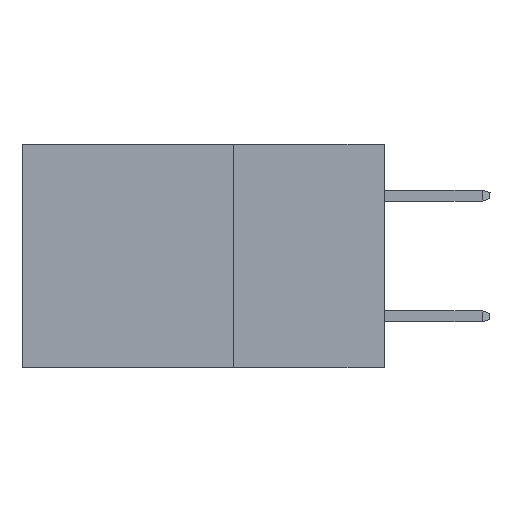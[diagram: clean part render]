
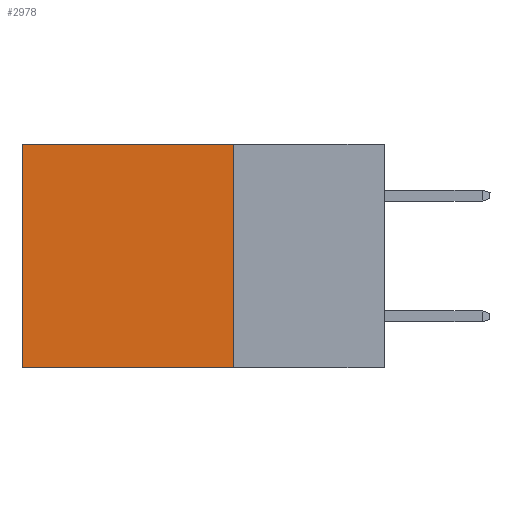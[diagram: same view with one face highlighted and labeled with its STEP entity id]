
A CAD part, left-side view. The second image highlights one B-rep face of the part: STEP entity #2978.
In plain terms, the highlighted planar face has unit normal (-1, 0, 0).
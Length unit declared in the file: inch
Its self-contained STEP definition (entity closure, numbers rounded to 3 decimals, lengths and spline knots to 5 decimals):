
#99 = CARTESIAN_POINT ( 'NONE',  ( 0.298, 0.25, 0. ) ) ;
#419 = LINE ( 'NONE', #7611, #7452 ) ;
#645 = CARTESIAN_POINT ( 'NONE',  ( 0.298, 0.25, 0. ) ) ;
#1768 = VERTEX_POINT ( 'NONE', #3185 ) ;
#1789 = ORIENTED_EDGE ( 'NONE', *, *, #9869, .T. ) ;
#1862 = EDGE_LOOP ( 'NONE', ( #8539, #2027, #6897, #1789 ) ) ;
#2027 = ORIENTED_EDGE ( 'NONE', *, *, #9769, .F. ) ;
#2496 = VERTEX_POINT ( 'NONE', #11890 ) ;
#2853 = VECTOR ( 'NONE', #11882, 39.37008 ) ;
#2978 = ADVANCED_FACE ( 'NONE', ( #3039 ), #5462, .F. ) ;
#3039 = FACE_OUTER_BOUND ( 'NONE', #1862, .T. ) ;
#3185 = CARTESIAN_POINT ( 'NONE',  ( 0.298, 0.6, 0. ) ) ;
#3239 = AXIS2_PLACEMENT_3D ( 'NONE', #10466, #12295, #11440 ) ;
#3275 = VECTOR ( 'NONE', #4026, 39.37008 ) ;
#3678 = EDGE_CURVE ( 'NONE', #7967, #11707, #419, .T. ) ;
#3906 = CARTESIAN_POINT ( 'NONE',  ( 0.298, 0.25, -0.37 ) ) ;
#4026 = DIRECTION ( 'NONE',  ( 0., 1., 0. ) ) ;
#4044 = EDGE_CURVE ( 'NONE', #1768, #2496, #8504, .T. ) ;
#5062 = CARTESIAN_POINT ( 'NONE',  ( 0.298, 0.6, 0. ) ) ;
#5462 = PLANE ( 'NONE',  #3239 ) ;
#5889 = LINE ( 'NONE', #99, #3275 ) ;
#6509 = DIRECTION ( 'NONE',  ( 0., 0., -1. ) ) ;
#6897 = ORIENTED_EDGE ( 'NONE', *, *, #3678, .F. ) ;
#7452 = VECTOR ( 'NONE', #6509, 39.37008 ) ;
#7611 = CARTESIAN_POINT ( 'NONE',  ( 0.298, 0.25, 0. ) ) ;
#7876 = VECTOR ( 'NONE', #11328, 39.37008 ) ;
#7967 = VERTEX_POINT ( 'NONE', #645 ) ;
#8504 = LINE ( 'NONE', #5062, #2853 ) ;
#8539 = ORIENTED_EDGE ( 'NONE', *, *, #4044, .T. ) ;
#9769 = EDGE_CURVE ( 'NONE', #11707, #2496, #11850, .T. ) ;
#9869 = EDGE_CURVE ( 'NONE', #7967, #1768, #5889, .T. ) ;
#10400 = CARTESIAN_POINT ( 'NONE',  ( 0.298, 0.25, -0.37 ) ) ;
#10466 = CARTESIAN_POINT ( 'NONE',  ( 0.298, 0.25, 0. ) ) ;
#11328 = DIRECTION ( 'NONE',  ( 0., 1., 0. ) ) ;
#11440 = DIRECTION ( 'NONE',  ( 0., 0., -1. ) ) ;
#11707 = VERTEX_POINT ( 'NONE', #3906 ) ;
#11850 = LINE ( 'NONE', #10400, #7876 ) ;
#11882 = DIRECTION ( 'NONE',  ( 0., 0., -1. ) ) ;
#11890 = CARTESIAN_POINT ( 'NONE',  ( 0.298, 0.6, -0.37 ) ) ;
#12295 = DIRECTION ( 'NONE',  ( 1., 0., 0. ) ) ;
